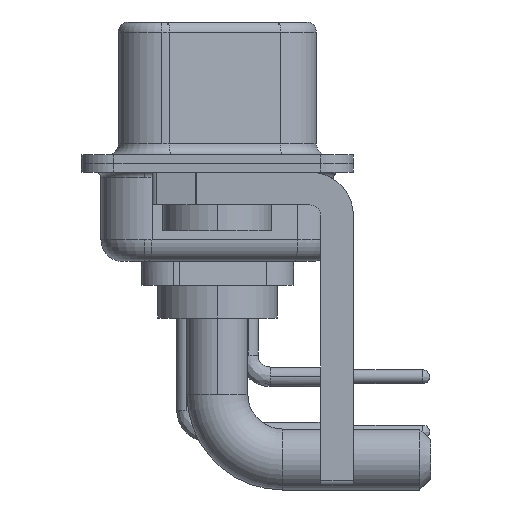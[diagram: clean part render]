
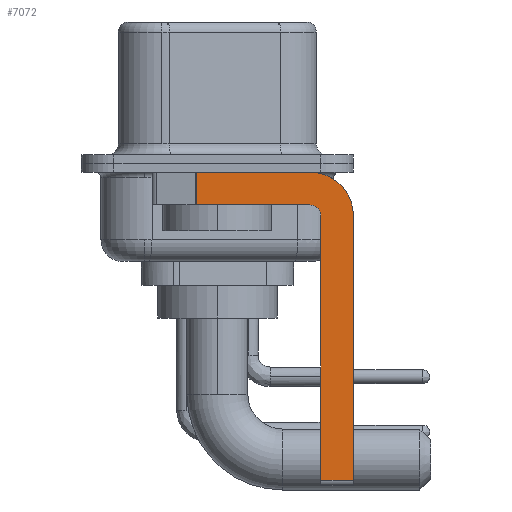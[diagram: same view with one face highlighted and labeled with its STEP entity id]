
A CAD part, left-side view. The second image highlights one B-rep face of the part: STEP entity #7072.
In plain terms, the highlighted planar face has unit normal (-1, 0, 0).
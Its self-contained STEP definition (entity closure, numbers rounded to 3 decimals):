
#289 = VERTEX_POINT ( 'NONE', #16878 ) ;
#339 = ORIENTED_EDGE ( 'NONE', *, *, #25356, .F. ) ;
#1162 = DIRECTION ( 'NONE',  ( 0., 0., -1. ) ) ;
#1436 = VECTOR ( 'NONE', #13719, 1000. ) ;
#1475 = CARTESIAN_POINT ( 'NONE',  ( -2.9, 3., -0.4 ) ) ;
#1731 = EDGE_CURVE ( 'NONE', #8259, #12381, #27112, .T. ) ;
#3590 = CARTESIAN_POINT ( 'NONE',  ( -2.9, 0.978, -1.9 ) ) ;
#4660 = VECTOR ( 'NONE', #17025, 1000. ) ;
#4968 = VERTEX_POINT ( 'NONE', #6350 ) ;
#5858 = LINE ( 'NONE', #8099, #27585 ) ;
#6350 = CARTESIAN_POINT ( 'NONE',  ( -2.9, -4.75, -2.4 ) ) ;
#7072 = ADVANCED_FACE ( 'NONE', ( #12449 ), #23356, .F. ) ;
#7503 = EDGE_LOOP ( 'NONE', ( #339, #18088, #24984, #16453, #26480, #15696, #18349, #24836 ) ) ;
#7592 = DIRECTION ( 'NONE',  ( 0., 0., -1. ) ) ;
#7760 = AXIS2_PLACEMENT_3D ( 'NONE', #16506, #21002, #12576 ) ;
#8099 = CARTESIAN_POINT ( 'NONE',  ( -2.9, 0.978, -1.9 ) ) ;
#8259 = VERTEX_POINT ( 'NONE', #25452 ) ;
#9197 = AXIS2_PLACEMENT_3D ( 'NONE', #22766, #24439, #1162 ) ;
#9869 = AXIS2_PLACEMENT_3D ( 'NONE', #27466, #25082, #16835 ) ;
#10452 = VERTEX_POINT ( 'NONE', #13479 ) ;
#10643 = CARTESIAN_POINT ( 'NONE',  ( -2.9, -4.25, -14.55 ) ) ;
#11015 = DIRECTION ( 'NONE',  ( 0., 0., -1. ) ) ;
#11886 = CIRCLE ( 'NONE', #9197, 2. ) ;
#12381 = VERTEX_POINT ( 'NONE', #3590 ) ;
#12449 = FACE_OUTER_BOUND ( 'NONE', #7503, .T. ) ;
#12576 = DIRECTION ( 'NONE',  ( 0., 0., -1. ) ) ;
#13479 = CARTESIAN_POINT ( 'NONE',  ( -2.9, -4.25, -0.4 ) ) ;
#13540 = VECTOR ( 'NONE', #20133, 1000. ) ;
#13719 = DIRECTION ( 'NONE',  ( 0., -1., 0. ) ) ;
#13733 = EDGE_CURVE ( 'NONE', #21592, #19569, #21314, .T. ) ;
#14358 = CARTESIAN_POINT ( 'NONE',  ( -2.9, -4.25, -1.9 ) ) ;
#14766 = CIRCLE ( 'NONE', #9869, 0.5 ) ;
#15469 = EDGE_CURVE ( 'NONE', #10452, #27413, #11886, .T. ) ;
#15696 = ORIENTED_EDGE ( 'NONE', *, *, #13733, .T. ) ;
#16453 = ORIENTED_EDGE ( 'NONE', *, *, #26776, .F. ) ;
#16471 = LINE ( 'NONE', #25002, #13540 ) ;
#16506 = CARTESIAN_POINT ( 'NONE',  ( -2.9, -4.25, -2.4 ) ) ;
#16835 = DIRECTION ( 'NONE',  ( 0., 0., 1. ) ) ;
#16878 = CARTESIAN_POINT ( 'NONE',  ( -2.9, 0.978, -0.4 ) ) ;
#17025 = DIRECTION ( 'NONE',  ( 0., 1., 0. ) ) ;
#18072 = LINE ( 'NONE', #1475, #1436 ) ;
#18088 = ORIENTED_EDGE ( 'NONE', *, *, #18339, .T. ) ;
#18339 = EDGE_CURVE ( 'NONE', #289, #12381, #5858, .T. ) ;
#18349 = ORIENTED_EDGE ( 'NONE', *, *, #26624, .F. ) ;
#19191 = DIRECTION ( 'NONE',  ( 0., -1., 0. ) ) ;
#19569 = VERTEX_POINT ( 'NONE', #24391 ) ;
#20133 = DIRECTION ( 'NONE',  ( 0., 0., 1. ) ) ;
#21002 = DIRECTION ( 'NONE',  ( 1., 0., 0. ) ) ;
#21314 = LINE ( 'NONE', #10643, #25847 ) ;
#21558 = CARTESIAN_POINT ( 'NONE',  ( -2.9, -4.75, -14.55 ) ) ;
#21592 = VERTEX_POINT ( 'NONE', #21558 ) ;
#22742 = LINE ( 'NONE', #24954, #23446 ) ;
#22766 = CARTESIAN_POINT ( 'NONE',  ( -2.9, -4.25, -2.4 ) ) ;
#23304 = EDGE_CURVE ( 'NONE', #21592, #4968, #16471, .T. ) ;
#23356 = PLANE ( 'NONE',  #7760 ) ;
#23446 = VECTOR ( 'NONE', #7592, 1000. ) ;
#23920 = CARTESIAN_POINT ( 'NONE',  ( -2.9, -6.25, -2.4 ) ) ;
#24391 = CARTESIAN_POINT ( 'NONE',  ( -2.9, -6.25, -14.55 ) ) ;
#24439 = DIRECTION ( 'NONE',  ( 1., 0., 0. ) ) ;
#24836 = ORIENTED_EDGE ( 'NONE', *, *, #15469, .F. ) ;
#24954 = CARTESIAN_POINT ( 'NONE',  ( -2.9, -6.25, -2.4 ) ) ;
#24984 = ORIENTED_EDGE ( 'NONE', *, *, #1731, .F. ) ;
#25002 = CARTESIAN_POINT ( 'NONE',  ( -2.9, -4.75, -14.8 ) ) ;
#25082 = DIRECTION ( 'NONE',  ( -1., 0., 0. ) ) ;
#25356 = EDGE_CURVE ( 'NONE', #289, #10452, #18072, .T. ) ;
#25452 = CARTESIAN_POINT ( 'NONE',  ( -2.9, -4.25, -1.9 ) ) ;
#25847 = VECTOR ( 'NONE', #19191, 1000. ) ;
#26480 = ORIENTED_EDGE ( 'NONE', *, *, #23304, .F. ) ;
#26624 = EDGE_CURVE ( 'NONE', #27413, #19569, #22742, .T. ) ;
#26776 = EDGE_CURVE ( 'NONE', #4968, #8259, #14766, .T. ) ;
#27112 = LINE ( 'NONE', #14358, #4660 ) ;
#27413 = VERTEX_POINT ( 'NONE', #23920 ) ;
#27466 = CARTESIAN_POINT ( 'NONE',  ( -2.9, -4.25, -2.4 ) ) ;
#27585 = VECTOR ( 'NONE', #11015, 1000. ) ;
